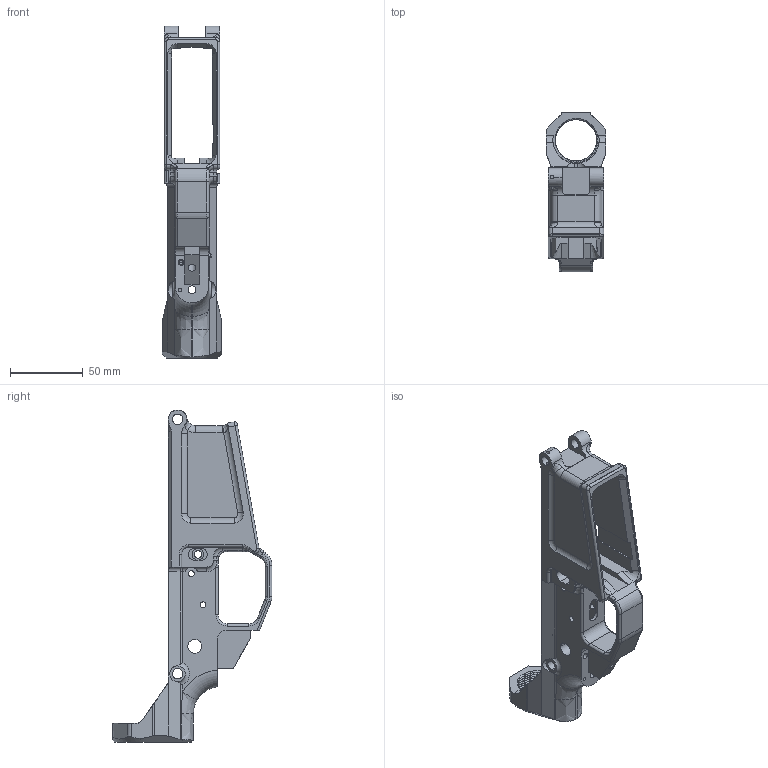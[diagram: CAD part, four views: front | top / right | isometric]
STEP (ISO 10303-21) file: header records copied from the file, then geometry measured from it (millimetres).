
FILE_DESCRIPTION (( 'STEP AP214' ), '1' );
FILE_NAME ('WX LOWER.STEP', '2016-04-23T06:01:17', ( '' ), ( '' ), 'SwSTEP 2.0', 'SolidWorks 2013', '' );
FILE_SCHEMA (( 'AUTOMOTIVE_DESIGN' ));
Length unit declared in the file: inch
Products named in the file (1): WX LOWER
Bounding box: 40.64 x 109.71 x 227.84 mm (x, y, z)
Volume: 130952.7 mm3; surface area: 62840.7 mm2
Topology: 1 solids, 4 shells, 445 faces, 1209 edges, 760 vertices
Faces by surface type: cylinder 192, plane 142, torus 58, bspline 38, cone 13, sphere 2
Entity records: 17809 total; most frequent: CARTESIAN_POINT 6867, ORIENTED_EDGE 2406, DIRECTION 2200, EDGE_CURVE 1203, AXIS2_PLACEMENT_3D 829, VERTEX_POINT 760, VECTOR 542, LINE 542
